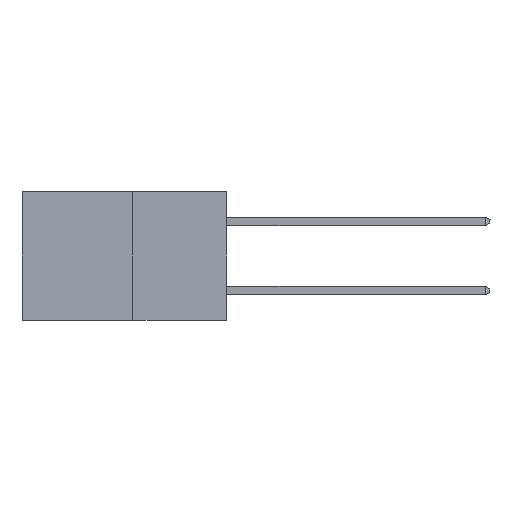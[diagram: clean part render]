
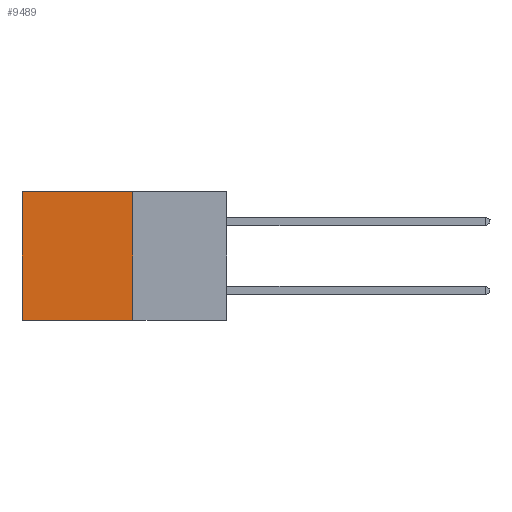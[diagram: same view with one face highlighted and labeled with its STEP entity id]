
A CAD part, left-side view. The second image highlights one B-rep face of the part: STEP entity #9489.
In plain terms, the highlighted planar face has unit normal (-1, 0, 0).
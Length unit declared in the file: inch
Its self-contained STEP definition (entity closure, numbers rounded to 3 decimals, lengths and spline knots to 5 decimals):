
#91 = EDGE_CURVE ( 'NONE', #8736, #1694, #2301, .T. ) ;
#522 = EDGE_CURVE ( 'NONE', #8736, #6689, #3004, .T. ) ;
#782 = ORIENTED_EDGE ( 'NONE', *, *, #4908, .T. ) ;
#1088 = CARTESIAN_POINT ( 'NONE',  ( 0.277, 0.27, 0. ) ) ;
#1427 = LINE ( 'NONE', #4071, #4147 ) ;
#1502 = CARTESIAN_POINT ( 'NONE',  ( 0.277, 0.27, -0.37 ) ) ;
#1694 = VERTEX_POINT ( 'NONE', #5957 ) ;
#1813 = DIRECTION ( 'NONE',  ( 0., 0., -1. ) ) ;
#2301 = LINE ( 'NONE', #3986, #8339 ) ;
#2440 = VERTEX_POINT ( 'NONE', #10101 ) ;
#2667 = DIRECTION ( 'NONE',  ( 0., 0., -1. ) ) ;
#3004 = LINE ( 'NONE', #1088, #14537 ) ;
#3986 = CARTESIAN_POINT ( 'NONE',  ( 0.277, 0.27, -0.37 ) ) ;
#4071 = CARTESIAN_POINT ( 'NONE',  ( 0.277, 0.27, -0.37 ) ) ;
#4147 = VECTOR ( 'NONE', #14117, 39.37008 ) ;
#4256 = CARTESIAN_POINT ( 'NONE',  ( 0.277, 0.59, -0.37 ) ) ;
#4556 = DIRECTION ( 'NONE',  ( 0., 0., -1. ) ) ;
#4908 = EDGE_CURVE ( 'NONE', #6689, #2440, #9511, .T. ) ;
#5162 = AXIS2_PLACEMENT_3D ( 'NONE', #1502, #9456, #2667 ) ;
#5719 = ORIENTED_EDGE ( 'NONE', *, *, #522, .T. ) ;
#5957 = CARTESIAN_POINT ( 'NONE',  ( 0.277, 0.27, -0.37 ) ) ;
#6347 = CARTESIAN_POINT ( 'NONE',  ( 0.277, 0.59, 0. ) ) ;
#6399 = ORIENTED_EDGE ( 'NONE', *, *, #91, .F. ) ;
#6689 = VERTEX_POINT ( 'NONE', #6347 ) ;
#6716 = DIRECTION ( 'NONE',  ( 0., 1., 0. ) ) ;
#7242 = PLANE ( 'NONE',  #5162 ) ;
#7283 = EDGE_LOOP ( 'NONE', ( #782, #8608, #6399, #5719 ) ) ;
#8339 = VECTOR ( 'NONE', #1813, 39.37008 ) ;
#8608 = ORIENTED_EDGE ( 'NONE', *, *, #10323, .F. ) ;
#8736 = VERTEX_POINT ( 'NONE', #12452 ) ;
#9456 = DIRECTION ( 'NONE',  ( 1., 0., 0. ) ) ;
#9489 = ADVANCED_FACE ( 'NONE', ( #12090 ), #7242, .F. ) ;
#9511 = LINE ( 'NONE', #4256, #12148 ) ;
#10101 = CARTESIAN_POINT ( 'NONE',  ( 0.277, 0.59, -0.37 ) ) ;
#10323 = EDGE_CURVE ( 'NONE', #1694, #2440, #1427, .T. ) ;
#12090 = FACE_OUTER_BOUND ( 'NONE', #7283, .T. ) ;
#12148 = VECTOR ( 'NONE', #4556, 39.37008 ) ;
#12452 = CARTESIAN_POINT ( 'NONE',  ( 0.277, 0.27, 0. ) ) ;
#14117 = DIRECTION ( 'NONE',  ( 0., 1., 0. ) ) ;
#14537 = VECTOR ( 'NONE', #6716, 39.37008 ) ;
